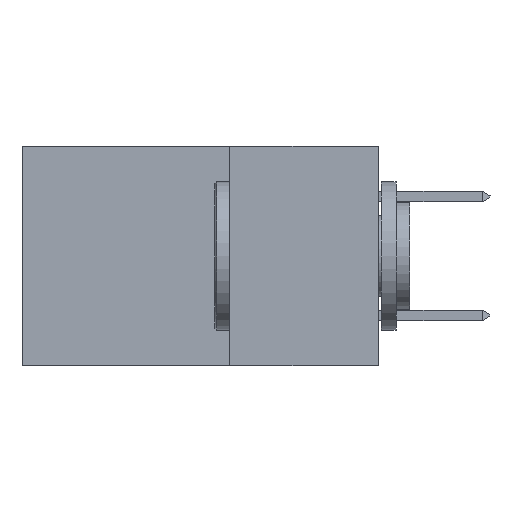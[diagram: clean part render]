
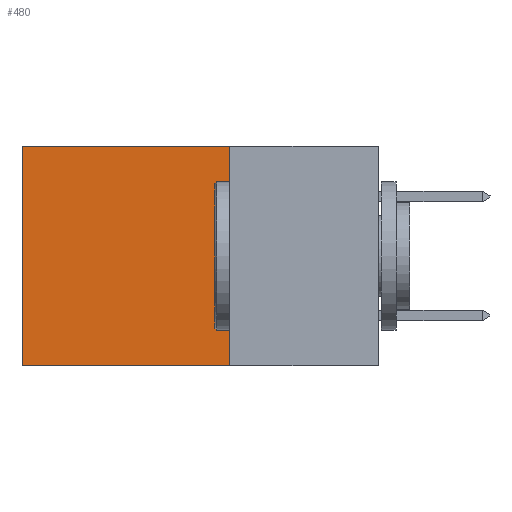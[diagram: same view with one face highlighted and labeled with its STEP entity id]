
A CAD part, left-side view. The second image highlights one B-rep face of the part: STEP entity #480.
In plain terms, the highlighted planar face has unit normal (-1, 0, 0).
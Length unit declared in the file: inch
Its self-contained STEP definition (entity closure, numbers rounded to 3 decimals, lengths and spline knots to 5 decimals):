
#244 = CARTESIAN_POINT ( 'NONE',  ( 0.2615, 0.25, -0.37 ) ) ;
#480 = ADVANCED_FACE ( 'NONE', ( #10562 ), #3086, .F. ) ;
#1088 = EDGE_CURVE ( 'NONE', #9263, #2194, #7472, .T. ) ;
#1994 = CARTESIAN_POINT ( 'NONE',  ( 0.2615, 0.6, -0.37 ) ) ;
#2194 = VERTEX_POINT ( 'NONE', #6195 ) ;
#2467 = VECTOR ( 'NONE', #18614, 39.37008 ) ;
#2751 = ORIENTED_EDGE ( 'NONE', *, *, #18173, .F. ) ;
#3086 = PLANE ( 'NONE',  #5990 ) ;
#4139 = CARTESIAN_POINT ( 'NONE',  ( 0.2615, 0.25, -0.37 ) ) ;
#4206 = EDGE_LOOP ( 'NONE', ( #23374, #22025, #2751, #14051 ) ) ;
#4378 = DIRECTION ( 'NONE',  ( 0., 1., 0. ) ) ;
#4537 = VECTOR ( 'NONE', #23391, 39.37008 ) ;
#4900 = DIRECTION ( 'NONE',  ( 1., 0., 0. ) ) ;
#5942 = VERTEX_POINT ( 'NONE', #13593 ) ;
#5990 = AXIS2_PLACEMENT_3D ( 'NONE', #15824, #4900, #23132 ) ;
#6098 = EDGE_CURVE ( 'NONE', #2194, #14717, #17872, .T. ) ;
#6175 = LINE ( 'NONE', #4139, #14606 ) ;
#6195 = CARTESIAN_POINT ( 'NONE',  ( 0.2615, 0.6, 0. ) ) ;
#6861 = CARTESIAN_POINT ( 'NONE',  ( 0.2615, 0.25, 0. ) ) ;
#7472 = LINE ( 'NONE', #13017, #2467 ) ;
#9263 = VERTEX_POINT ( 'NONE', #6861 ) ;
#10418 = EDGE_CURVE ( 'NONE', #5942, #14717, #6175, .T. ) ;
#10562 = FACE_OUTER_BOUND ( 'NONE', #4206, .T. ) ;
#13017 = CARTESIAN_POINT ( 'NONE',  ( 0.2615, 0.25, 0. ) ) ;
#13593 = CARTESIAN_POINT ( 'NONE',  ( 0.2615, 0.25, -0.37 ) ) ;
#14051 = ORIENTED_EDGE ( 'NONE', *, *, #1088, .T. ) ;
#14531 = CARTESIAN_POINT ( 'NONE',  ( 0.2615, 0.6, -0.37 ) ) ;
#14606 = VECTOR ( 'NONE', #4378, 39.37008 ) ;
#14717 = VERTEX_POINT ( 'NONE', #1994 ) ;
#15824 = CARTESIAN_POINT ( 'NONE',  ( 0.2615, 0.25, -0.37 ) ) ;
#17872 = LINE ( 'NONE', #14531, #4537 ) ;
#18173 = EDGE_CURVE ( 'NONE', #9263, #5942, #22099, .T. ) ;
#18377 = DIRECTION ( 'NONE',  ( 0., 0., -1. ) ) ;
#18614 = DIRECTION ( 'NONE',  ( 0., 1., 0. ) ) ;
#20850 = VECTOR ( 'NONE', #18377, 39.37008 ) ;
#22025 = ORIENTED_EDGE ( 'NONE', *, *, #10418, .F. ) ;
#22099 = LINE ( 'NONE', #244, #20850 ) ;
#23132 = DIRECTION ( 'NONE',  ( 0., 0., -1. ) ) ;
#23374 = ORIENTED_EDGE ( 'NONE', *, *, #6098, .T. ) ;
#23391 = DIRECTION ( 'NONE',  ( 0., 0., -1. ) ) ;
